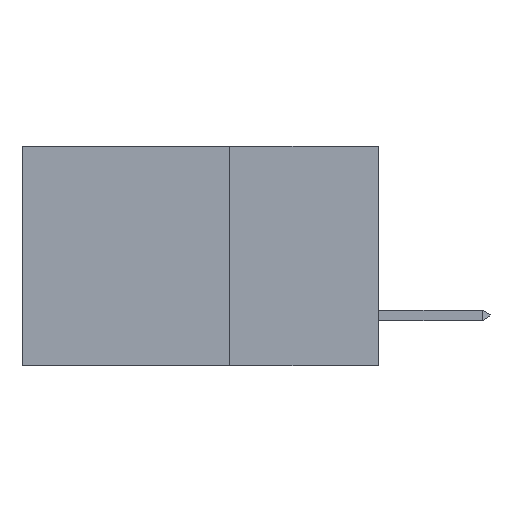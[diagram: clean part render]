
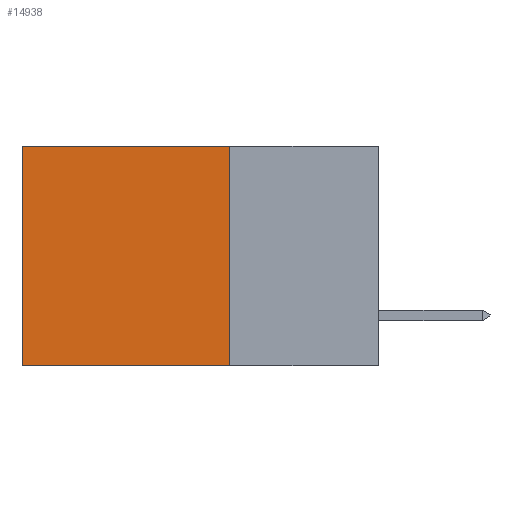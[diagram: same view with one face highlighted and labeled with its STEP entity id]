
A CAD part, left-side view. The second image highlights one B-rep face of the part: STEP entity #14938.
In plain terms, the highlighted planar face has unit normal (-1, 0, 0).
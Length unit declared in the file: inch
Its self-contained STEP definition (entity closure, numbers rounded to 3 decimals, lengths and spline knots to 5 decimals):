
#641 = DIRECTION ( 'NONE',  ( 0., 1., 0. ) ) ;
#997 = DIRECTION ( 'NONE',  ( 0., 1., 0. ) ) ;
#1069 = VERTEX_POINT ( 'NONE', #13296 ) ;
#1124 = ORIENTED_EDGE ( 'NONE', *, *, #6098, .F. ) ;
#1264 = EDGE_CURVE ( 'NONE', #14706, #15097, #12442, .T. ) ;
#1592 = LINE ( 'NONE', #11034, #8556 ) ;
#2211 = VECTOR ( 'NONE', #12740, 39.37008 ) ;
#2388 = DIRECTION ( 'NONE',  ( 0., 0., -1. ) ) ;
#2677 = CARTESIAN_POINT ( 'NONE',  ( 0.298, 0.25, 0. ) ) ;
#3261 = FACE_OUTER_BOUND ( 'NONE', #3721, .T. ) ;
#3721 = EDGE_LOOP ( 'NONE', ( #5848, #1124, #6788, #11653 ) ) ;
#4163 = PLANE ( 'NONE',  #10489 ) ;
#4530 = CARTESIAN_POINT ( 'NONE',  ( 0.298, 0.25, 0. ) ) ;
#4741 = EDGE_CURVE ( 'NONE', #14706, #8201, #1592, .T. ) ;
#5498 = VECTOR ( 'NONE', #641, 39.37008 ) ;
#5848 = ORIENTED_EDGE ( 'NONE', *, *, #5855, .T. ) ;
#5855 = EDGE_CURVE ( 'NONE', #15097, #1069, #15852, .T. ) ;
#6098 = EDGE_CURVE ( 'NONE', #8201, #1069, #8774, .T. ) ;
#6788 = ORIENTED_EDGE ( 'NONE', *, *, #4741, .F. ) ;
#7100 = CARTESIAN_POINT ( 'NONE',  ( 0.298, 0.25, -0.37 ) ) ;
#7504 = VECTOR ( 'NONE', #997, 39.37008 ) ;
#8201 = VERTEX_POINT ( 'NONE', #15889 ) ;
#8556 = VECTOR ( 'NONE', #2388, 39.37008 ) ;
#8774 = LINE ( 'NONE', #7100, #5498 ) ;
#10059 = DIRECTION ( 'NONE',  ( 1., 0., 0. ) ) ;
#10489 = AXIS2_PLACEMENT_3D ( 'NONE', #2677, #10059, #11253 ) ;
#11034 = CARTESIAN_POINT ( 'NONE',  ( 0.298, 0.25, 0. ) ) ;
#11253 = DIRECTION ( 'NONE',  ( 0., 0., -1. ) ) ;
#11653 = ORIENTED_EDGE ( 'NONE', *, *, #1264, .T. ) ;
#12119 = CARTESIAN_POINT ( 'NONE',  ( 0.298, 0.25, 0. ) ) ;
#12401 = CARTESIAN_POINT ( 'NONE',  ( 0.298, 0.6, 0. ) ) ;
#12442 = LINE ( 'NONE', #4530, #7504 ) ;
#12672 = CARTESIAN_POINT ( 'NONE',  ( 0.298, 0.6, 0. ) ) ;
#12740 = DIRECTION ( 'NONE',  ( 0., 0., -1. ) ) ;
#13296 = CARTESIAN_POINT ( 'NONE',  ( 0.298, 0.6, -0.37 ) ) ;
#14706 = VERTEX_POINT ( 'NONE', #12119 ) ;
#14938 = ADVANCED_FACE ( 'NONE', ( #3261 ), #4163, .F. ) ;
#15097 = VERTEX_POINT ( 'NONE', #12401 ) ;
#15852 = LINE ( 'NONE', #12672, #2211 ) ;
#15889 = CARTESIAN_POINT ( 'NONE',  ( 0.298, 0.25, -0.37 ) ) ;
